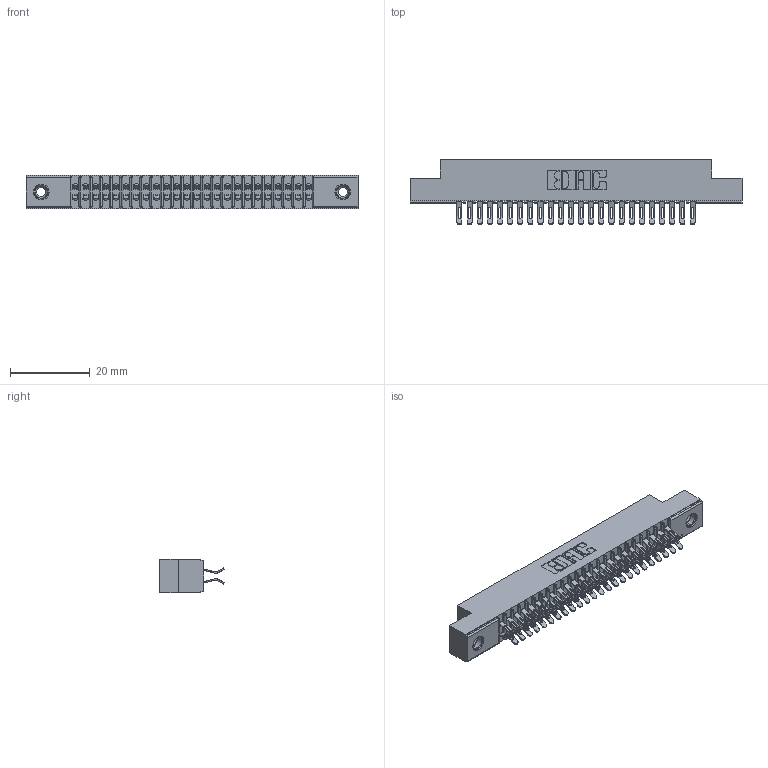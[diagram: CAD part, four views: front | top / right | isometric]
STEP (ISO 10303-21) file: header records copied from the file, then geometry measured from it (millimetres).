
FILE_DESCRIPTION (( 'STEP AP203' ), '1' );
FILE_NAME ('341-048-555-208.STEP', '2018-08-07T11:54:58', ( '' ), ( '' ), 'SwSTEP 2.0', 'SolidWorks 2016', '' );
FILE_SCHEMA (( 'CONFIG_CONTROL_DESIGN' ));
Length unit declared in the file: inch
Products named in the file (4): 341 Part_.156 (3.96) Dia Mounting Holes; 341-292-001_341-292-155; 345-250-001_345-250-003-102; 341-048-555-208
Assembly tree (51 placements, depth 2):
  341-048-555-208
    341 Part_.156 (3.96) Dia Mounting Holes
    341-292-001_341-292-155  x48
    345-250-001_345-250-003-102  x2
Bounding box: 83.19 x 16.31 x 8.38 mm (x, y, z)
Volume: 4784.9 mm3; surface area: 10482.5 mm2
Topology: 51 solids, 51 shells, 3920 faces, 11660 edges, 7586 vertices
Faces by surface type: plane 2116, cylinder 1692, sphere 50, torus 50, cone 12
Entity records: 33098 total; most frequent: CARTESIAN_POINT 5501, ORIENTED_EDGE 5448, DIRECTION 5352, EDGE_CURVE 2724, LINE 2162, VECTOR 2162, VERTEX_POINT 1728, AXIS2_PLACEMENT_3D 1595
